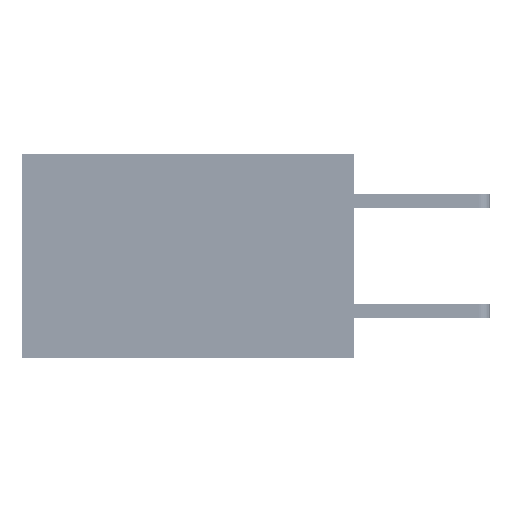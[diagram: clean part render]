
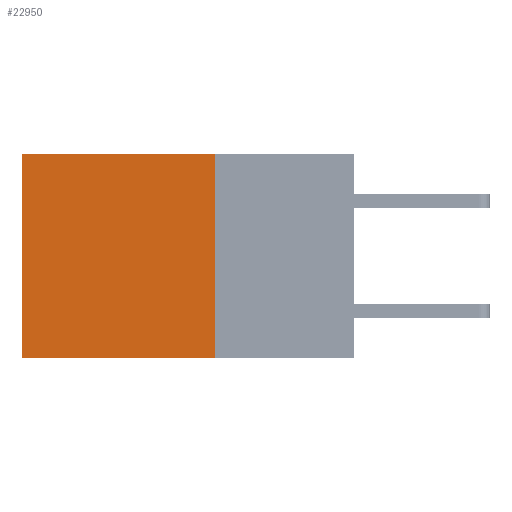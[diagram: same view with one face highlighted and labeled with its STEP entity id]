
A CAD part, left-side view. The second image highlights one B-rep face of the part: STEP entity #22950.
In plain terms, the highlighted planar face has unit normal (-1, 0, 0).
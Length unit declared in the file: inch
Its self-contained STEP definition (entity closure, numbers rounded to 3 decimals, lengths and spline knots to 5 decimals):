
#31 = CARTESIAN_POINT ( 'NONE',  ( 0.2875, 0.25, 0. ) ) ;
#86 = DIRECTION ( 'NONE',  ( 0., 0., -1. ) ) ;
#801 = CARTESIAN_POINT ( 'NONE',  ( 0.2875, 0.25, 0. ) ) ;
#1138 = EDGE_CURVE ( 'NONE', #36406, #25152, #38164, .T. ) ;
#4048 = EDGE_CURVE ( 'NONE', #36406, #25944, #35116, .T. ) ;
#6241 = EDGE_CURVE ( 'NONE', #25944, #18696, #33135, .T. ) ;
#8200 = VECTOR ( 'NONE', #35847, 39.37008 ) ;
#9215 = DIRECTION ( 'NONE',  ( 0., 1., 0. ) ) ;
#9642 = ORIENTED_EDGE ( 'NONE', *, *, #4048, .T. ) ;
#11158 = CARTESIAN_POINT ( 'NONE',  ( 0.2875, 0.25, -0.37 ) ) ;
#11512 = DIRECTION ( 'NONE',  ( 1., 0., 0. ) ) ;
#13774 = LINE ( 'NONE', #28286, #42768 ) ;
#15457 = ORIENTED_EDGE ( 'NONE', *, *, #1138, .F. ) ;
#15537 = AXIS2_PLACEMENT_3D ( 'NONE', #801, #11512, #86 ) ;
#16647 = ORIENTED_EDGE ( 'NONE', *, *, #6241, .T. ) ;
#18696 = VERTEX_POINT ( 'NONE', #32209 ) ;
#19127 = PLANE ( 'NONE',  #15537 ) ;
#20837 = CARTESIAN_POINT ( 'NONE',  ( 0.2875, 0.25, 0. ) ) ;
#21568 = CARTESIAN_POINT ( 'NONE',  ( 0.2875, 0.6, 0. ) ) ;
#22950 = ADVANCED_FACE ( 'NONE', ( #32910 ), #19127, .F. ) ;
#25152 = VERTEX_POINT ( 'NONE', #11158 ) ;
#25944 = VERTEX_POINT ( 'NONE', #31702 ) ;
#28160 = ORIENTED_EDGE ( 'NONE', *, *, #44360, .F. ) ;
#28286 = CARTESIAN_POINT ( 'NONE',  ( 0.2875, 0.25, -0.37 ) ) ;
#30452 = EDGE_LOOP ( 'NONE', ( #16647, #28160, #15457, #9642 ) ) ;
#31702 = CARTESIAN_POINT ( 'NONE',  ( 0.2875, 0.6, 0. ) ) ;
#32209 = CARTESIAN_POINT ( 'NONE',  ( 0.2875, 0.6, -0.37 ) ) ;
#32910 = FACE_OUTER_BOUND ( 'NONE', #30452, .T. ) ;
#33135 = LINE ( 'NONE', #21568, #8200 ) ;
#33251 = VECTOR ( 'NONE', #9215, 39.37008 ) ;
#34103 = CARTESIAN_POINT ( 'NONE',  ( 0.2875, 0.25, 0. ) ) ;
#35116 = LINE ( 'NONE', #20837, #33251 ) ;
#35847 = DIRECTION ( 'NONE',  ( 0., 0., -1. ) ) ;
#36406 = VERTEX_POINT ( 'NONE', #31 ) ;
#38164 = LINE ( 'NONE', #34103, #39494 ) ;
#39494 = VECTOR ( 'NONE', #45049, 39.37008 ) ;
#42768 = VECTOR ( 'NONE', #42789, 39.37008 ) ;
#42789 = DIRECTION ( 'NONE',  ( 0., 1., 0. ) ) ;
#44360 = EDGE_CURVE ( 'NONE', #25152, #18696, #13774, .T. ) ;
#45049 = DIRECTION ( 'NONE',  ( 0., 0., -1. ) ) ;
